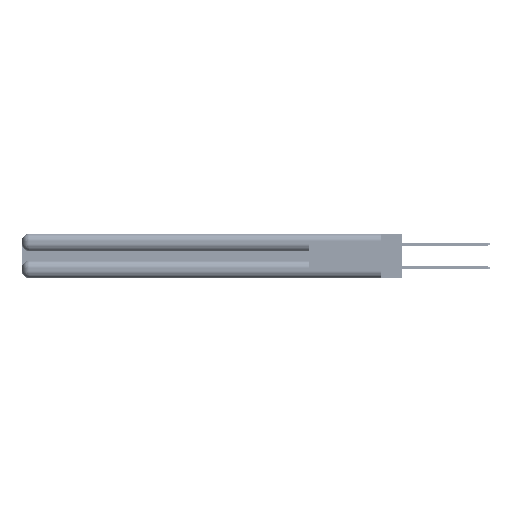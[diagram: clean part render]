
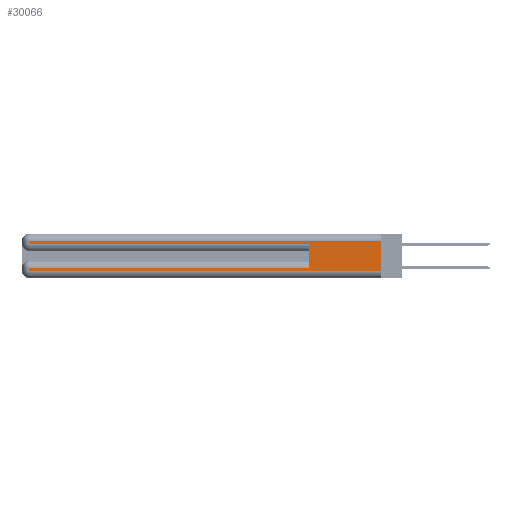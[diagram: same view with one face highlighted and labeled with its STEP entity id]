
A CAD part, left-side view. The second image highlights one B-rep face of the part: STEP entity #30066.
In plain terms, the highlighted planar face has unit normal (-1, 0, 0).
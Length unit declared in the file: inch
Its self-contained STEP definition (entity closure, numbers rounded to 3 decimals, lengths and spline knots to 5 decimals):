
#75 = DIRECTION ( 'NONE',  ( 0., 0., -1. ) ) ;
#339 = VERTEX_POINT ( 'NONE', #42434 ) ;
#1767 = VERTEX_POINT ( 'NONE', #55859 ) ;
#3073 = LINE ( 'NONE', #57123, #49191 ) ;
#3168 = LINE ( 'NONE', #17662, #24225 ) ;
#3909 = LINE ( 'NONE', #19675, #14451 ) ;
#4196 = ORIENTED_EDGE ( 'NONE', *, *, #50521, .F. ) ;
#5709 = ORIENTED_EDGE ( 'NONE', *, *, #53943, .F. ) ;
#6320 = CARTESIAN_POINT ( 'NONE',  ( 0., 0.6, 0.145 ) ) ;
#7480 = ORIENTED_EDGE ( 'NONE', *, *, #46135, .T. ) ;
#7638 = PLANE ( 'NONE',  #45292 ) ;
#7811 = ORIENTED_EDGE ( 'NONE', *, *, #22587, .T. ) ;
#8351 = CARTESIAN_POINT ( 'NONE',  ( 0., 0.6, 0.285 ) ) ;
#9439 = VECTOR ( 'NONE', #19830, 39.37008 ) ;
#10154 = FACE_OUTER_BOUND ( 'NONE', #26697, .T. ) ;
#10794 = LINE ( 'NONE', #36924, #56809 ) ;
#10934 = EDGE_CURVE ( 'NONE', #30714, #11690, #51941, .T. ) ;
#11061 = DIRECTION ( 'NONE',  ( 0., -1., 0. ) ) ;
#11690 = VERTEX_POINT ( 'NONE', #30190 ) ;
#12990 = VERTEX_POINT ( 'NONE', #8351 ) ;
#13610 = VECTOR ( 'NONE', #50167, 39.37008 ) ;
#14451 = VECTOR ( 'NONE', #11061, 39.37008 ) ;
#17003 = CARTESIAN_POINT ( 'NONE',  ( 0., 0.6, 0.085 ) ) ;
#17314 = ORIENTED_EDGE ( 'NONE', *, *, #25272, .T. ) ;
#17662 = CARTESIAN_POINT ( 'NONE',  ( 0., 2.94, 0.37 ) ) ;
#19675 = CARTESIAN_POINT ( 'NONE',  ( 0., 0., 0.06 ) ) ;
#19830 = DIRECTION ( 'NONE',  ( 0., 0., 1. ) ) ;
#21144 = CARTESIAN_POINT ( 'NONE',  ( 0., 0., 0.37 ) ) ;
#21813 = ORIENTED_EDGE ( 'NONE', *, *, #10934, .T. ) ;
#22453 = CARTESIAN_POINT ( 'NONE',  ( 0., 0., 0.37 ) ) ;
#22587 = EDGE_CURVE ( 'NONE', #339, #12990, #10794, .T. ) ;
#22643 = ORIENTED_EDGE ( 'NONE', *, *, #47943, .T. ) ;
#23463 = DIRECTION ( 'NONE',  ( 0., -1., 0. ) ) ;
#24035 = ORIENTED_EDGE ( 'NONE', *, *, #49021, .T. ) ;
#24225 = VECTOR ( 'NONE', #39885, 39.37008 ) ;
#25272 = EDGE_CURVE ( 'NONE', #28078, #339, #3168, .T. ) ;
#25640 = VERTEX_POINT ( 'NONE', #51064 ) ;
#25677 = DIRECTION ( 'NONE',  ( 0., 0., -1. ) ) ;
#26697 = EDGE_LOOP ( 'NONE', ( #5709, #7480, #17314, #7811, #4196, #21813, #22643, #24035 ) ) ;
#26742 = VECTOR ( 'NONE', #57523, 39.37008 ) ;
#28078 = VERTEX_POINT ( 'NONE', #50968 ) ;
#30066 = ADVANCED_FACE ( 'NONE', ( #10154 ), #7638, .F. ) ;
#30190 = CARTESIAN_POINT ( 'NONE',  ( 0., 2.94, 0.085 ) ) ;
#30714 = VERTEX_POINT ( 'NONE', #17003 ) ;
#34959 = VERTEX_POINT ( 'NONE', #42568 ) ;
#36039 = LINE ( 'NONE', #6320, #9439 ) ;
#36924 = CARTESIAN_POINT ( 'NONE',  ( 0., 0., 0.285 ) ) ;
#39500 = DIRECTION ( 'NONE',  ( 0., 1., 0. ) ) ;
#39885 = DIRECTION ( 'NONE',  ( 0., 0., -1. ) ) ;
#42434 = CARTESIAN_POINT ( 'NONE',  ( 0., 2.94, 0.285 ) ) ;
#42551 = VECTOR ( 'NONE', #75, 39.37008 ) ;
#42568 = CARTESIAN_POINT ( 'NONE',  ( 0., 2.94, 0.06 ) ) ;
#45292 = AXIS2_PLACEMENT_3D ( 'NONE', #21144, #52267, #25677 ) ;
#45741 = CARTESIAN_POINT ( 'NONE',  ( 0., 0., 0.085 ) ) ;
#46135 = EDGE_CURVE ( 'NONE', #1767, #28078, #3073, .T. ) ;
#47943 = EDGE_CURVE ( 'NONE', #11690, #34959, #51757, .T. ) ;
#49021 = EDGE_CURVE ( 'NONE', #34959, #25640, #3909, .T. ) ;
#49191 = VECTOR ( 'NONE', #39500, 39.37008 ) ;
#50167 = DIRECTION ( 'NONE',  ( 0., 1., 0. ) ) ;
#50521 = EDGE_CURVE ( 'NONE', #30714, #12990, #36039, .T. ) ;
#50968 = CARTESIAN_POINT ( 'NONE',  ( 0., 2.94, 0.31 ) ) ;
#51064 = CARTESIAN_POINT ( 'NONE',  ( 0., 0., 0.06 ) ) ;
#51757 = LINE ( 'NONE', #53074, #26742 ) ;
#51941 = LINE ( 'NONE', #45741, #13610 ) ;
#52267 = DIRECTION ( 'NONE',  ( 1., 0., 0. ) ) ;
#53074 = CARTESIAN_POINT ( 'NONE',  ( 0., 2.94, 0.37 ) ) ;
#53943 = EDGE_CURVE ( 'NONE', #1767, #25640, #54347, .T. ) ;
#54347 = LINE ( 'NONE', #22453, #42551 ) ;
#55859 = CARTESIAN_POINT ( 'NONE',  ( 0., 0., 0.31 ) ) ;
#56809 = VECTOR ( 'NONE', #23463, 39.37008 ) ;
#57123 = CARTESIAN_POINT ( 'NONE',  ( 0., 0., 0.31 ) ) ;
#57523 = DIRECTION ( 'NONE',  ( 0., 0., -1. ) ) ;
